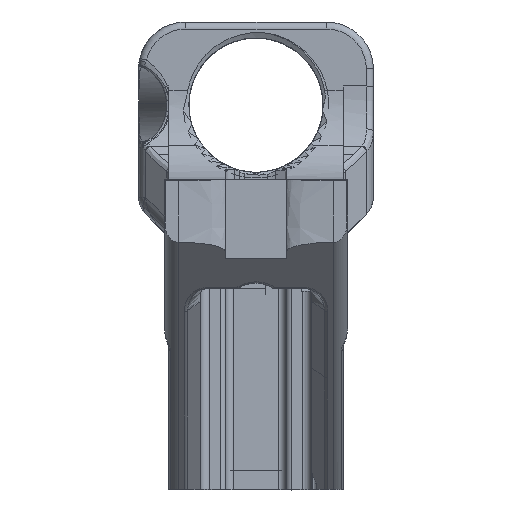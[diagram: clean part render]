
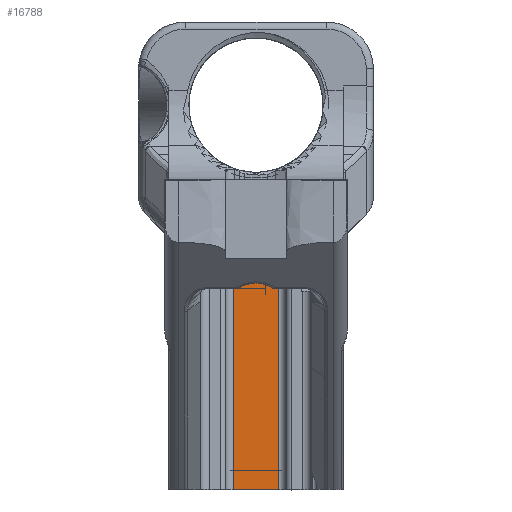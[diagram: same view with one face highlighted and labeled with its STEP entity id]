
A CAD part, top view. The second image highlights one B-rep face of the part: STEP entity #16788.
In plain terms, the highlighted planar face has unit normal (0, 0, 1).
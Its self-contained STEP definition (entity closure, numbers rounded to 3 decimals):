
#654 = ORIENTED_EDGE ( 'NONE', *, *, #15935, .T. ) ;
#922 = CARTESIAN_POINT ( 'NONE',  ( -15.45, -62.864, 115.839 ) ) ;
#2808 = CARTESIAN_POINT ( 'NONE',  ( -5.797, -62.864, 115.839 ) ) ;
#3841 = PLANE ( 'NONE',  #35066 ) ;
#5216 = CARTESIAN_POINT ( 'NONE',  ( -15.45, 2.926, 115.839 ) ) ;
#5703 = DIRECTION ( 'NONE',  ( 0., -1., 0. ) ) ;
#5991 = CARTESIAN_POINT ( 'NONE',  ( -15.45, -62.864, 115.839 ) ) ;
#6860 = CARTESIAN_POINT ( 'NONE',  ( 7.973, 2.926, 115.839 ) ) ;
#8260 = VERTEX_POINT ( 'NONE', #2808 ) ;
#8295 = VECTOR ( 'NONE', #5703, 1000. ) ;
#9501 = DIRECTION ( 'NONE',  ( 0., 0., -1. ) ) ;
#10993 = CARTESIAN_POINT ( 'NONE',  ( -5.797, -62.864, 115.839 ) ) ;
#11727 = EDGE_LOOP ( 'NONE', ( #35646, #35355, #27408, #654 ) ) ;
#12082 = FACE_OUTER_BOUND ( 'NONE', #11727, .T. ) ;
#12168 = CARTESIAN_POINT ( 'NONE',  ( -15.45, -19.004, 115.839 ) ) ;
#12573 = CARTESIAN_POINT ( 'NONE',  ( -10.623, -62.864, 115.839 ) ) ;
#15059 = DIRECTION ( 'NONE',  ( -1., 0., 0. ) ) ;
#15578 = EDGE_CURVE ( 'NONE', #8260, #23819, #34798, .T. ) ;
#15935 = EDGE_CURVE ( 'NONE', #19562, #34836, #24391, .T. ) ;
#16788 = ADVANCED_FACE ( 'NONE', ( #12082 ), #3841, .F. ) ;
#19358 = EDGE_CURVE ( 'NONE', #19562, #8260, #28747, .T. ) ;
#19562 = VERTEX_POINT ( 'NONE', #23699 ) ;
#19702 = CARTESIAN_POINT ( 'NONE',  ( -15.45, 2.926, 115.839 ) ) ;
#20443 = CARTESIAN_POINT ( 'NONE',  ( -15.45, -40.934, 115.839 ) ) ;
#21751 = B_SPLINE_CURVE_WITH_KNOTS ( 'NONE', 3,
 ( #19702, #12168, #20443, #5991 ),
 .UNSPECIFIED., .F., .F.,
 ( 4, 4 ),
 ( 0., 1. ),
 .UNSPECIFIED. ) ;
#23699 = CARTESIAN_POINT ( 'NONE',  ( -5.797, 2.926, 115.839 ) ) ;
#23819 = VERTEX_POINT ( 'NONE', #922 ) ;
#24220 = EDGE_CURVE ( 'NONE', #34836, #23819, #21751, .T. ) ;
#24391 = LINE ( 'NONE', #6860, #32978 ) ;
#26371 = CARTESIAN_POINT ( 'NONE',  ( -23.339, -62.864, 115.839 ) ) ;
#27408 = ORIENTED_EDGE ( 'NONE', *, *, #19358, .F. ) ;
#27592 = VECTOR ( 'NONE', #15059, 1000. ) ;
#28747 = LINE ( 'NONE', #10993, #8295 ) ;
#29818 = DIRECTION ( 'NONE',  ( 0., -1., 0. ) ) ;
#29933 = DIRECTION ( 'NONE',  ( -1., 0., 0. ) ) ;
#32978 = VECTOR ( 'NONE', #29933, 1000. ) ;
#34798 = LINE ( 'NONE', #26371, #27592 ) ;
#34836 = VERTEX_POINT ( 'NONE', #5216 ) ;
#35066 = AXIS2_PLACEMENT_3D ( 'NONE', #12573, #9501, #29818 ) ;
#35355 = ORIENTED_EDGE ( 'NONE', *, *, #15578, .F. ) ;
#35646 = ORIENTED_EDGE ( 'NONE', *, *, #24220, .T. ) ;
